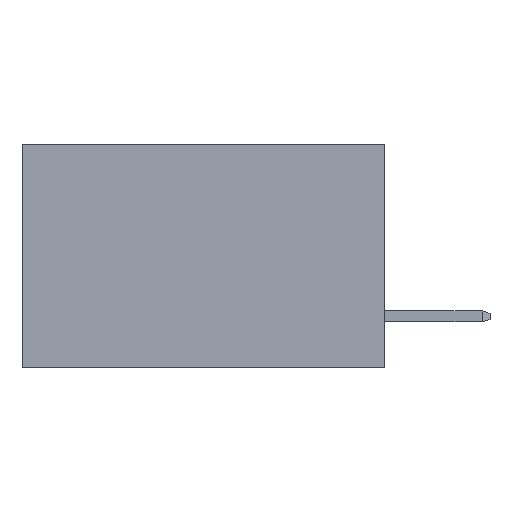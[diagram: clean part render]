
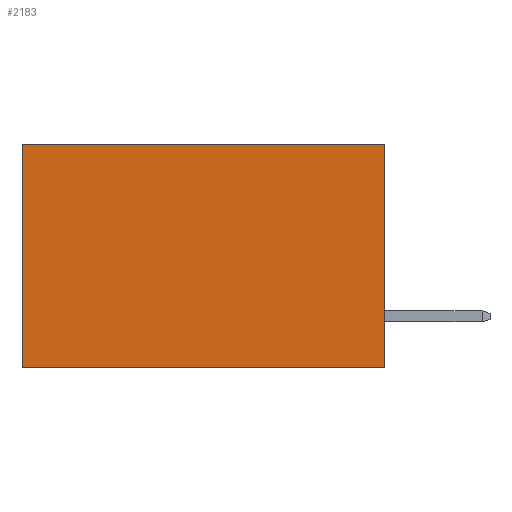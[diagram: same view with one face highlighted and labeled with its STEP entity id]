
A CAD part, left-side view. The second image highlights one B-rep face of the part: STEP entity #2183.
In plain terms, the highlighted planar face has unit normal (-1, 0, 0).
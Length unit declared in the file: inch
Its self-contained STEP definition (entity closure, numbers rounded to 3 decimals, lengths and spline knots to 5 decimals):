
#220 = VECTOR ( 'NONE', #9208, 39.37008 ) ;
#337 = EDGE_CURVE ( 'NONE', #9909, #759, #2808, .T. ) ;
#553 = LINE ( 'NONE', #10019, #8075 ) ;
#738 = CARTESIAN_POINT ( 'NONE',  ( 0.298, 0., 0. ) ) ;
#759 = VERTEX_POINT ( 'NONE', #1738 ) ;
#1005 = ORIENTED_EDGE ( 'NONE', *, *, #337, .F. ) ;
#1098 = EDGE_CURVE ( 'NONE', #9909, #10292, #6054, .T. ) ;
#1711 = PLANE ( 'NONE',  #10372 ) ;
#1738 = CARTESIAN_POINT ( 'NONE',  ( 0.298, 0., -0.37 ) ) ;
#1784 = DIRECTION ( 'NONE',  ( 0., 1., 0. ) ) ;
#2183 = ADVANCED_FACE ( 'NONE', ( #7697 ), #1711, .F. ) ;
#2329 = ORIENTED_EDGE ( 'NONE', *, *, #4234, .F. ) ;
#2808 = LINE ( 'NONE', #3637, #220 ) ;
#2982 = ORIENTED_EDGE ( 'NONE', *, *, #5285, .T. ) ;
#3537 = VECTOR ( 'NONE', #1784, 39.37008 ) ;
#3637 = CARTESIAN_POINT ( 'NONE',  ( 0.298, 0., 0. ) ) ;
#4234 = EDGE_CURVE ( 'NONE', #759, #8990, #4977, .T. ) ;
#4587 = DIRECTION ( 'NONE',  ( 0., 0., -1. ) ) ;
#4622 = DIRECTION ( 'NONE',  ( 1., 0., 0. ) ) ;
#4821 = DIRECTION ( 'NONE',  ( 0., 1., 0. ) ) ;
#4977 = LINE ( 'NONE', #8457, #6835 ) ;
#5285 = EDGE_CURVE ( 'NONE', #10292, #8990, #553, .T. ) ;
#6054 = LINE ( 'NONE', #738, #3537 ) ;
#6138 = ORIENTED_EDGE ( 'NONE', *, *, #1098, .T. ) ;
#6835 = VECTOR ( 'NONE', #4821, 39.37008 ) ;
#7205 = CARTESIAN_POINT ( 'NONE',  ( 0.298, 0.6, 0. ) ) ;
#7697 = FACE_OUTER_BOUND ( 'NONE', #10526, .T. ) ;
#8075 = VECTOR ( 'NONE', #4587, 39.37008 ) ;
#8199 = CARTESIAN_POINT ( 'NONE',  ( 0.298, 0.6, -0.37 ) ) ;
#8457 = CARTESIAN_POINT ( 'NONE',  ( 0.298, 0., -0.37 ) ) ;
#8990 = VERTEX_POINT ( 'NONE', #8199 ) ;
#9208 = DIRECTION ( 'NONE',  ( 0., 0., -1. ) ) ;
#9391 = CARTESIAN_POINT ( 'NONE',  ( 0.298, 0., 0. ) ) ;
#9909 = VERTEX_POINT ( 'NONE', #9391 ) ;
#10019 = CARTESIAN_POINT ( 'NONE',  ( 0.298, 0.6, 0. ) ) ;
#10292 = VERTEX_POINT ( 'NONE', #7205 ) ;
#10372 = AXIS2_PLACEMENT_3D ( 'NONE', #11420, #4622, #11455 ) ;
#10526 = EDGE_LOOP ( 'NONE', ( #2982, #2329, #1005, #6138 ) ) ;
#11420 = CARTESIAN_POINT ( 'NONE',  ( 0.298, 0., 0. ) ) ;
#11455 = DIRECTION ( 'NONE',  ( 0., 0., -1. ) ) ;
